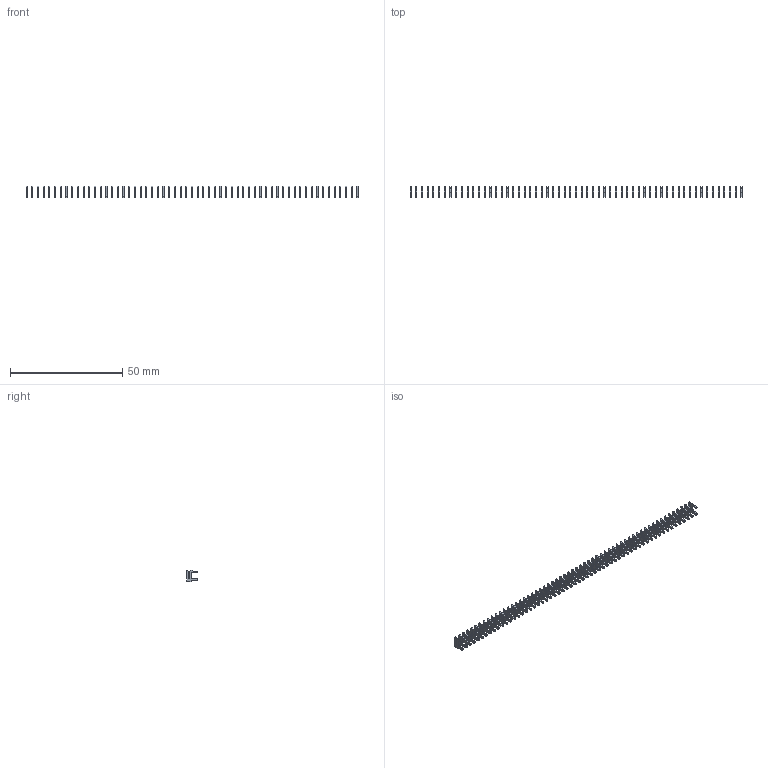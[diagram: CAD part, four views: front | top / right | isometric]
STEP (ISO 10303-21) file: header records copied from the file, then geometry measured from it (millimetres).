
FILE_DESCRIPTION (( 'STEP AP203' ), '1' );
FILE_NAME ('105-059-208-100.STEP', '2020-04-08T00:54:04', ( '' ), ( '' ), 'SwSTEP 2.0', 'SolidWorks 2016', '' );
FILE_SCHEMA (( 'CONFIG_CONTROL_DESIGN' ));
Length unit declared in the file: inch
Products named in the file (2): 105-059-208-100; 100-290-001_100-290-208
Assembly tree (59 placements, depth 2):
  105-059-208-100
    100-290-001_100-290-208  x59
Bounding box: 147.83 x 4.83 x 5.17 mm (x, y, z)
Volume: 406 mm3; surface area: 2507.3 mm2
Topology: 59 solids, 59 shells, 1475 faces, 4071 edges, 2714 vertices
Faces by surface type: plane 1298, cylinder 177
Entity records: 2845 total; most frequent: DIRECTION 249, CARTESIAN_POINT 202, ORIENTED_EDGE 138, LOCAL_TIME 128, CALENDAR_DATE 128, COORDINATED_UNIVERSAL_TIME_OFFSET 128, DATE_AND_TIME 128, AXIS2_PLACEMENT_3D 93
